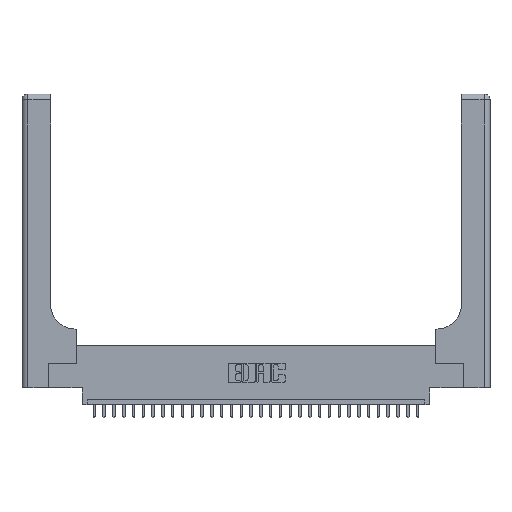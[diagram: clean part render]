
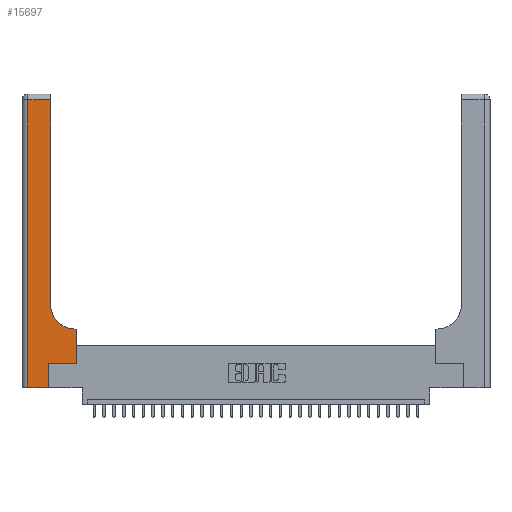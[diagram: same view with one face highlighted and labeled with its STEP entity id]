
A CAD part, top view. The second image highlights one B-rep face of the part: STEP entity #15697.
In plain terms, the highlighted planar face has unit normal (0, 0, 1).
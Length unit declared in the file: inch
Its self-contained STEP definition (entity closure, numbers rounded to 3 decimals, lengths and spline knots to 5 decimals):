
#12 = DIRECTION ( 'NONE',  ( -1., 0., 0. ) ) ;
#114 = CARTESIAN_POINT ( 'NONE',  ( 0.06, 0., 0.37 ) ) ;
#875 = LINE ( 'NONE', #13386, #14341 ) ;
#935 = EDGE_CURVE ( 'NONE', #23148, #26450, #29605, .T. ) ;
#1821 = VERTEX_POINT ( 'NONE', #17600 ) ;
#2040 = CARTESIAN_POINT ( 'NONE',  ( 0.5585, 0.6, 0.37 ) ) ;
#2137 = DIRECTION ( 'NONE',  ( 0., 1., 0. ) ) ;
#2353 = VECTOR ( 'NONE', #30921, 39.37008 ) ;
#2789 = VERTEX_POINT ( 'NONE', #18910 ) ;
#3166 = EDGE_CURVE ( 'NONE', #19433, #23148, #875, .T. ) ;
#3194 = CARTESIAN_POINT ( 'NONE',  ( 0., 3., 0.37 ) ) ;
#3345 = EDGE_CURVE ( 'NONE', #12450, #26709, #22082, .T. ) ;
#3429 = EDGE_CURVE ( 'NONE', #26709, #1821, #31365, .T. ) ;
#4498 = CARTESIAN_POINT ( 'NONE',  ( 0.2915, 3., 0.37 ) ) ;
#5867 = LINE ( 'NONE', #7222, #8572 ) ;
#5938 = DIRECTION ( 'NONE',  ( 0., 1., 0. ) ) ;
#6058 = DIRECTION ( 'NONE',  ( 1., 0., 0. ) ) ;
#6964 = ORIENTED_EDGE ( 'NONE', *, *, #3345, .T. ) ;
#7222 = CARTESIAN_POINT ( 'NONE',  ( 0.269, 0.25, 0.37 ) ) ;
#7408 = CARTESIAN_POINT ( 'NONE',  ( 0.269, 0., 0.37 ) ) ;
#7503 = AXIS2_PLACEMENT_3D ( 'NONE', #8758, #13909, #6058 ) ;
#7628 = VECTOR ( 'NONE', #12, 39.37008 ) ;
#8119 = LINE ( 'NONE', #16787, #23544 ) ;
#8421 = CARTESIAN_POINT ( 'NONE',  ( 0.5585, 0.25, 0.37 ) ) ;
#8431 = DIRECTION ( 'NONE',  ( 1., 0., 0. ) ) ;
#8572 = VECTOR ( 'NONE', #24266, 39.37008 ) ;
#8758 = CARTESIAN_POINT ( 'NONE',  ( 0.5415, 0.85, 0.37 ) ) ;
#10762 = ORIENTED_EDGE ( 'NONE', *, *, #935, .T. ) ;
#10966 = CARTESIAN_POINT ( 'NONE',  ( 0.2915, 0.85, 0.37 ) ) ;
#11032 = CARTESIAN_POINT ( 'NONE',  ( 0.5415, 0.6, 0.37 ) ) ;
#12450 = VERTEX_POINT ( 'NONE', #11032 ) ;
#13194 = ORIENTED_EDGE ( 'NONE', *, *, #31017, .T. ) ;
#13234 = DIRECTION ( 'NONE',  ( 0., 0., -1. ) ) ;
#13320 = CARTESIAN_POINT ( 'NONE',  ( 0.06, 3., 0.37 ) ) ;
#13386 = CARTESIAN_POINT ( 'NONE',  ( 0., 0., 0.37 ) ) ;
#13909 = DIRECTION ( 'NONE',  ( 0., 0., -1. ) ) ;
#14181 = DIRECTION ( 'NONE',  ( -1., 0., 0. ) ) ;
#14341 = VECTOR ( 'NONE', #8431, 39.37008 ) ;
#14469 = ORIENTED_EDGE ( 'NONE', *, *, #14913, .T. ) ;
#14783 = CARTESIAN_POINT ( 'NONE',  ( 0.2915, 0.6, 0.37 ) ) ;
#14913 = EDGE_CURVE ( 'NONE', #26450, #2789, #5867, .T. ) ;
#15697 = ADVANCED_FACE ( 'NONE', ( #17806 ), #17961, .F. ) ;
#15927 = DIRECTION ( 'NONE',  ( -1., 0., 0. ) ) ;
#16787 = CARTESIAN_POINT ( 'NONE',  ( 0., 2.94, 0.37 ) ) ;
#17179 = VECTOR ( 'NONE', #5938, 39.37008 ) ;
#17600 = CARTESIAN_POINT ( 'NONE',  ( 0.2915, 2.94, 0.37 ) ) ;
#17806 = FACE_OUTER_BOUND ( 'NONE', #23175, .T. ) ;
#17961 = PLANE ( 'NONE',  #19499 ) ;
#18447 = ORIENTED_EDGE ( 'NONE', *, *, #3429, .T. ) ;
#18593 = VECTOR ( 'NONE', #2137, 39.37008 ) ;
#18910 = CARTESIAN_POINT ( 'NONE',  ( 0.5585, 0.25, 0.37 ) ) ;
#19216 = VERTEX_POINT ( 'NONE', #2040 ) ;
#19433 = VERTEX_POINT ( 'NONE', #114 ) ;
#19499 = AXIS2_PLACEMENT_3D ( 'NONE', #3194, #13234, #15927 ) ;
#20537 = CARTESIAN_POINT ( 'NONE',  ( 0.06, 2.94, 0.37 ) ) ;
#21064 = ORIENTED_EDGE ( 'NONE', *, *, #22679, .T. ) ;
#22082 = CIRCLE ( 'NONE', #7503, 0.25 ) ;
#22679 = EDGE_CURVE ( 'NONE', #2789, #19216, #30333, .T. ) ;
#23017 = VECTOR ( 'NONE', #29220, 39.37008 ) ;
#23148 = VERTEX_POINT ( 'NONE', #27859 ) ;
#23175 = EDGE_LOOP ( 'NONE', ( #18447, #13194, #23547, #28486, #10762, #14469, #21064, #24728, #6964 ) ) ;
#23437 = LINE ( 'NONE', #14783, #7628 ) ;
#23544 = VECTOR ( 'NONE', #14181, 39.37008 ) ;
#23547 = ORIENTED_EDGE ( 'NONE', *, *, #28565, .T. ) ;
#24266 = DIRECTION ( 'NONE',  ( 1., 0., 0. ) ) ;
#24728 = ORIENTED_EDGE ( 'NONE', *, *, #24954, .T. ) ;
#24954 = EDGE_CURVE ( 'NONE', #19216, #12450, #23437, .T. ) ;
#25401 = CARTESIAN_POINT ( 'NONE',  ( 0.269, 0.25, 0.37 ) ) ;
#26450 = VERTEX_POINT ( 'NONE', #25401 ) ;
#26709 = VERTEX_POINT ( 'NONE', #10966 ) ;
#27859 = CARTESIAN_POINT ( 'NONE',  ( 0.269, 0., 0.37 ) ) ;
#28486 = ORIENTED_EDGE ( 'NONE', *, *, #3166, .T. ) ;
#28565 = EDGE_CURVE ( 'NONE', #31318, #19433, #30568, .T. ) ;
#29220 = DIRECTION ( 'NONE',  ( 0., 1., 0. ) ) ;
#29605 = LINE ( 'NONE', #7408, #23017 ) ;
#30333 = LINE ( 'NONE', #8421, #17179 ) ;
#30568 = LINE ( 'NONE', #13320, #2353 ) ;
#30921 = DIRECTION ( 'NONE',  ( 0., -1., 0. ) ) ;
#31017 = EDGE_CURVE ( 'NONE', #1821, #31318, #8119, .T. ) ;
#31318 = VERTEX_POINT ( 'NONE', #20537 ) ;
#31365 = LINE ( 'NONE', #4498, #18593 ) ;
